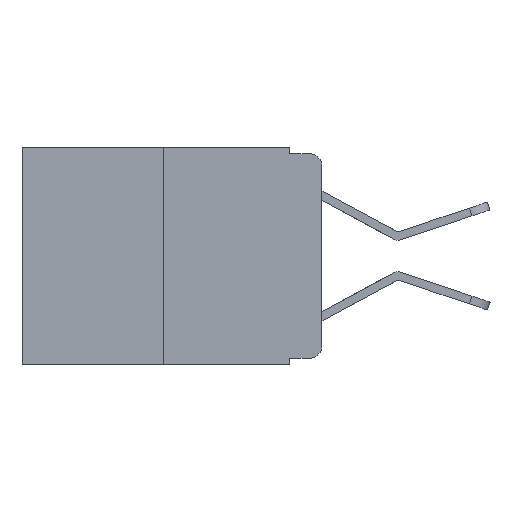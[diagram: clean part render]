
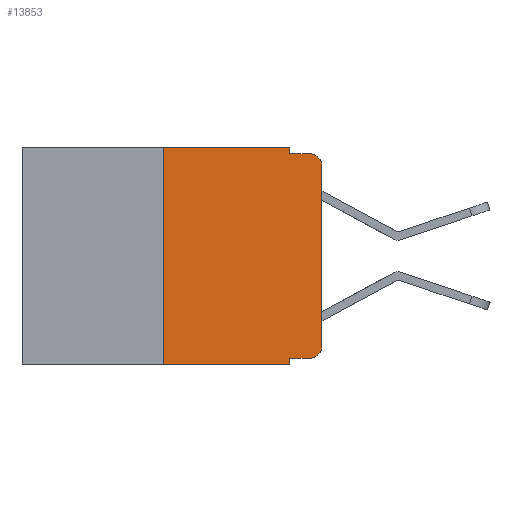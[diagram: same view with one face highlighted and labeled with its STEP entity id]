
A CAD part, left-side view. The second image highlights one B-rep face of the part: STEP entity #13853.
In plain terms, the highlighted planar face has unit normal (-1, 0, 0).
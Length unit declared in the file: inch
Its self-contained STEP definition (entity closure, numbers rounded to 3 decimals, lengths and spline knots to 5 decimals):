
#17 = CIRCLE ( 'NONE', #8608, 0.02 ) ;
#264 = CARTESIAN_POINT ( 'NONE',  ( 0., 0., -0.313 ) ) ;
#391 = VECTOR ( 'NONE', #2230, 39.37008 ) ;
#677 = ORIENTED_EDGE ( 'NONE', *, *, #13109, .T. ) ;
#693 = CARTESIAN_POINT ( 'NONE',  ( 0., 0.25, -0.343 ) ) ;
#816 = CARTESIAN_POINT ( 'NONE',  ( 0., 0.051, 0. ) ) ;
#831 = AXIS2_PLACEMENT_3D ( 'NONE', #2237, #4326, #12165 ) ;
#840 = DIRECTION ( 'NONE',  ( 0., 0., -1. ) ) ;
#947 = CARTESIAN_POINT ( 'NONE',  ( 0., 0.051, -0.333 ) ) ;
#1345 = VERTEX_POINT ( 'NONE', #264 ) ;
#1636 = ORIENTED_EDGE ( 'NONE', *, *, #1717, .F. ) ;
#1672 = CARTESIAN_POINT ( 'NONE',  ( 0., 0.25, 0. ) ) ;
#1717 = EDGE_CURVE ( 'NONE', #13418, #12785, #6203, .T. ) ;
#1925 = LINE ( 'NONE', #10230, #2610 ) ;
#1977 = CARTESIAN_POINT ( 'NONE',  ( 0., 0., 0. ) ) ;
#2230 = DIRECTION ( 'NONE',  ( 0., -1., 0. ) ) ;
#2237 = CARTESIAN_POINT ( 'NONE',  ( 0., 0.473, 0. ) ) ;
#2610 = VECTOR ( 'NONE', #8077, 39.37008 ) ;
#2778 = VERTEX_POINT ( 'NONE', #693 ) ;
#2819 = VERTEX_POINT ( 'NONE', #11476 ) ;
#2965 = DIRECTION ( 'NONE',  ( 0., -1., 0. ) ) ;
#2995 = DIRECTION ( 'NONE',  ( 0., 0., 1. ) ) ;
#3177 = VERTEX_POINT ( 'NONE', #6803 ) ;
#3227 = EDGE_CURVE ( 'NONE', #2819, #5212, #1925, .T. ) ;
#3276 = VERTEX_POINT ( 'NONE', #3587 ) ;
#3587 = CARTESIAN_POINT ( 'NONE',  ( 0., 0., -0.03 ) ) ;
#3710 = EDGE_CURVE ( 'NONE', #3276, #5212, #17, .T. ) ;
#4326 = DIRECTION ( 'NONE',  ( 1., 0., 0. ) ) ;
#4845 = EDGE_CURVE ( 'NONE', #8443, #5033, #12463, .T. ) ;
#5033 = VERTEX_POINT ( 'NONE', #10906 ) ;
#5041 = AXIS2_PLACEMENT_3D ( 'NONE', #11748, #13848, #8591 ) ;
#5051 = ORIENTED_EDGE ( 'NONE', *, *, #13016, .T. ) ;
#5174 = CARTESIAN_POINT ( 'NONE',  ( 0., 0.473, -0.343 ) ) ;
#5212 = VERTEX_POINT ( 'NONE', #11842 ) ;
#5342 = DIRECTION ( 'NONE',  ( -1., 0., 0. ) ) ;
#5721 = ORIENTED_EDGE ( 'NONE', *, *, #9645, .T. ) ;
#6088 = LINE ( 'NONE', #947, #14125 ) ;
#6203 = LINE ( 'NONE', #12247, #391 ) ;
#6266 = FACE_OUTER_BOUND ( 'NONE', #8033, .T. ) ;
#6533 = PLANE ( 'NONE',  #831 ) ;
#6803 = CARTESIAN_POINT ( 'NONE',  ( 0., 0.02, -0.333 ) ) ;
#7133 = VECTOR ( 'NONE', #12909, 39.37008 ) ;
#7442 = EDGE_CURVE ( 'NONE', #1345, #3276, #12953, .T. ) ;
#8033 = EDGE_LOOP ( 'NONE', ( #11003, #12304, #12201, #11234, #1636, #13473, #5721, #8602, #677, #5051 ) ) ;
#8077 = DIRECTION ( 'NONE',  ( 0., -1., 0. ) ) ;
#8443 = VERTEX_POINT ( 'NONE', #12087 ) ;
#8534 = DIRECTION ( 'NONE',  ( 0., 0., -1. ) ) ;
#8591 = DIRECTION ( 'NONE',  ( 0., 0., -1. ) ) ;
#8602 = ORIENTED_EDGE ( 'NONE', *, *, #4845, .F. ) ;
#8608 = AXIS2_PLACEMENT_3D ( 'NONE', #12988, #5342, #8534 ) ;
#9141 = EDGE_CURVE ( 'NONE', #2778, #13418, #10795, .T. ) ;
#9546 = VECTOR ( 'NONE', #840, 39.37008 ) ;
#9645 = EDGE_CURVE ( 'NONE', #2778, #5033, #12215, .T. ) ;
#10230 = CARTESIAN_POINT ( 'NONE',  ( 0., 0.051, -0.01 ) ) ;
#10369 = LINE ( 'NONE', #13923, #9546 ) ;
#10795 = LINE ( 'NONE', #12980, #11329 ) ;
#10906 = CARTESIAN_POINT ( 'NONE',  ( 0., 0.051, -0.343 ) ) ;
#11003 = ORIENTED_EDGE ( 'NONE', *, *, #7442, .T. ) ;
#11219 = CIRCLE ( 'NONE', #5041, 0.02 ) ;
#11234 = ORIENTED_EDGE ( 'NONE', *, *, #13661, .F. ) ;
#11329 = VECTOR ( 'NONE', #2995, 39.37008 ) ;
#11476 = CARTESIAN_POINT ( 'NONE',  ( 0., 0.051, -0.01 ) ) ;
#11748 = CARTESIAN_POINT ( 'NONE',  ( 0., 0.02, -0.313 ) ) ;
#11749 = DIRECTION ( 'NONE',  ( 0., 0., -1. ) ) ;
#11758 = DIRECTION ( 'NONE',  ( 0., -1., 0. ) ) ;
#11842 = CARTESIAN_POINT ( 'NONE',  ( 0., 0.02, -0.01 ) ) ;
#12087 = CARTESIAN_POINT ( 'NONE',  ( 0., 0.051, -0.333 ) ) ;
#12165 = DIRECTION ( 'NONE',  ( 0., 0., -1. ) ) ;
#12201 = ORIENTED_EDGE ( 'NONE', *, *, #3227, .F. ) ;
#12215 = LINE ( 'NONE', #5174, #12379 ) ;
#12247 = CARTESIAN_POINT ( 'NONE',  ( 0., 0.473, 0. ) ) ;
#12304 = ORIENTED_EDGE ( 'NONE', *, *, #3710, .T. ) ;
#12379 = VECTOR ( 'NONE', #11758, 39.37008 ) ;
#12463 = LINE ( 'NONE', #816, #12799 ) ;
#12785 = VERTEX_POINT ( 'NONE', #13484 ) ;
#12799 = VECTOR ( 'NONE', #11749, 39.37008 ) ;
#12909 = DIRECTION ( 'NONE',  ( 0., 0., 1. ) ) ;
#12953 = LINE ( 'NONE', #1977, #7133 ) ;
#12980 = CARTESIAN_POINT ( 'NONE',  ( 0., 0.25, 0. ) ) ;
#12988 = CARTESIAN_POINT ( 'NONE',  ( 0., 0.02, -0.03 ) ) ;
#13016 = EDGE_CURVE ( 'NONE', #3177, #1345, #11219, .T. ) ;
#13109 = EDGE_CURVE ( 'NONE', #8443, #3177, #6088, .T. ) ;
#13418 = VERTEX_POINT ( 'NONE', #1672 ) ;
#13473 = ORIENTED_EDGE ( 'NONE', *, *, #9141, .F. ) ;
#13484 = CARTESIAN_POINT ( 'NONE',  ( 0., 0.051, 0. ) ) ;
#13661 = EDGE_CURVE ( 'NONE', #12785, #2819, #10369, .T. ) ;
#13848 = DIRECTION ( 'NONE',  ( -1., 0., 0. ) ) ;
#13853 = ADVANCED_FACE ( 'NONE', ( #6266 ), #6533, .F. ) ;
#13923 = CARTESIAN_POINT ( 'NONE',  ( 0., 0.051, 0. ) ) ;
#14125 = VECTOR ( 'NONE', #2965, 39.37008 ) ;
